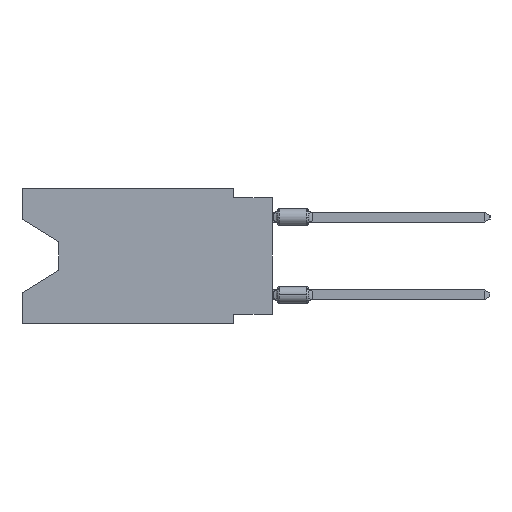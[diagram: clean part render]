
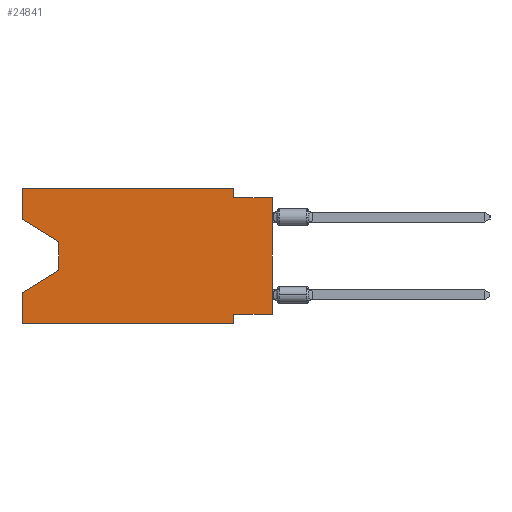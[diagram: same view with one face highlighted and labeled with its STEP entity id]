
A CAD part, left-side view. The second image highlights one B-rep face of the part: STEP entity #24841.
In plain terms, the highlighted planar face has unit normal (-1, 0, 0).
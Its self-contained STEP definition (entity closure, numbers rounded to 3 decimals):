
#209 = ORIENTED_EDGE ( 'NONE', *, *, #25861, .F. ) ;
#904 = VERTEX_POINT ( 'NONE', #20817 ) ;
#1866 = CARTESIAN_POINT ( 'NONE',  ( 0., 16.383, -8.89 ) ) ;
#4241 = CARTESIAN_POINT ( 'NONE',  ( 0., 13.97, -5.385 ) ) ;
#4389 = EDGE_CURVE ( 'NONE', #56818, #61978, #41734, .T. ) ;
#4486 = DIRECTION ( 'NONE',  ( 0., 0., -1. ) ) ;
#4579 = VECTOR ( 'NONE', #59693, 1000. ) ;
#4594 = VECTOR ( 'NONE', #38464, 1000. ) ;
#5525 = DIRECTION ( 'NONE',  ( 1., 0., 0. ) ) ;
#6193 = VECTOR ( 'NONE', #41860, 1000. ) ;
#6540 = VECTOR ( 'NONE', #58698, 1000. ) ;
#7580 = CARTESIAN_POINT ( 'NONE',  ( 0., 16.383, -6.852 ) ) ;
#8468 = VECTOR ( 'NONE', #64617, 1000. ) ;
#10137 = ORIENTED_EDGE ( 'NONE', *, *, #46131, .F. ) ;
#11813 = EDGE_CURVE ( 'NONE', #35556, #67885, #19351, .T. ) ;
#12263 = CARTESIAN_POINT ( 'NONE',  ( 0., 16.383, 0. ) ) ;
#12501 = VECTOR ( 'NONE', #23945, 1000. ) ;
#13232 = FACE_OUTER_BOUND ( 'NONE', #20999, .T. ) ;
#15757 = VERTEX_POINT ( 'NONE', #4241 ) ;
#15976 = CARTESIAN_POINT ( 'NONE',  ( 0., 16.383, -8.89 ) ) ;
#16066 = LINE ( 'NONE', #48453, #6193 ) ;
#17114 = EDGE_CURVE ( 'NONE', #15757, #41587, #45465, .T. ) ;
#17407 = EDGE_CURVE ( 'NONE', #61978, #28222, #37441, .T. ) ;
#17533 = CARTESIAN_POINT ( 'NONE',  ( 0., 13.97, -3.505 ) ) ;
#17977 = ORIENTED_EDGE ( 'NONE', *, *, #35410, .F. ) ;
#18123 = DIRECTION ( 'NONE',  ( 0., 0., 1. ) ) ;
#18981 = CARTESIAN_POINT ( 'NONE',  ( 0., 13.97, -5.385 ) ) ;
#19351 = LINE ( 'NONE', #20041, #64963 ) ;
#19603 = EDGE_CURVE ( 'NONE', #54139, #15757, #37781, .T. ) ;
#20041 = CARTESIAN_POINT ( 'NONE',  ( 0., 2.54, -8.89 ) ) ;
#20817 = CARTESIAN_POINT ( 'NONE',  ( 0., 16.383, -2.038 ) ) ;
#20999 = EDGE_LOOP ( 'NONE', ( #61478, #53809, #47068, #10137, #35614, #25546, #34554, #67553, #33373, #47545, #209, #17977 ) ) ;
#22217 = LINE ( 'NONE', #15976, #27086 ) ;
#23341 = CARTESIAN_POINT ( 'NONE',  ( 0., 16.383, 0. ) ) ;
#23405 = LINE ( 'NONE', #12263, #4579 ) ;
#23945 = DIRECTION ( 'NONE',  ( 0., 0., 1. ) ) ;
#24428 = VECTOR ( 'NONE', #49301, 1000. ) ;
#24841 = ADVANCED_FACE ( 'NONE', ( #13232 ), #34501, .F. ) ;
#25546 = ORIENTED_EDGE ( 'NONE', *, *, #11813, .F. ) ;
#25861 = EDGE_CURVE ( 'NONE', #46460, #56818, #27667, .T. ) ;
#26429 = VECTOR ( 'NONE', #62992, 1000. ) ;
#26431 = CARTESIAN_POINT ( 'NONE',  ( 0., 0., -0.635 ) ) ;
#27086 = VECTOR ( 'NONE', #38263, 1000. ) ;
#27667 = LINE ( 'NONE', #54495, #8468 ) ;
#28222 = VERTEX_POINT ( 'NONE', #26431 ) ;
#28438 = AXIS2_PLACEMENT_3D ( 'NONE', #47366, #5525, #4486 ) ;
#29304 = VERTEX_POINT ( 'NONE', #1866 ) ;
#29680 = CARTESIAN_POINT ( 'NONE',  ( 0., 13.97, -3.505 ) ) ;
#30039 = CARTESIAN_POINT ( 'NONE',  ( 0., 0., -8.255 ) ) ;
#30171 = EDGE_CURVE ( 'NONE', #52649, #28222, #50416, .T. ) ;
#30585 = CARTESIAN_POINT ( 'NONE',  ( 0., 2.54, 0. ) ) ;
#33373 = ORIENTED_EDGE ( 'NONE', *, *, #17407, .F. ) ;
#33531 = CARTESIAN_POINT ( 'NONE',  ( 0., 2.54, 0. ) ) ;
#34501 = PLANE ( 'NONE',  #28438 ) ;
#34554 = ORIENTED_EDGE ( 'NONE', *, *, #60709, .F. ) ;
#35410 = EDGE_CURVE ( 'NONE', #904, #46460, #23405, .T. ) ;
#35556 = VERTEX_POINT ( 'NONE', #62338 ) ;
#35614 = ORIENTED_EDGE ( 'NONE', *, *, #37666, .T. ) ;
#37237 = CARTESIAN_POINT ( 'NONE',  ( 0., 2.54, -8.89 ) ) ;
#37441 = LINE ( 'NONE', #68803, #6540 ) ;
#37666 = EDGE_CURVE ( 'NONE', #29304, #67885, #22217, .T. ) ;
#37713 = CARTESIAN_POINT ( 'NONE',  ( 0., 16.383, 0. ) ) ;
#37757 = CARTESIAN_POINT ( 'NONE',  ( 0., 2.54, -0.635 ) ) ;
#37781 = LINE ( 'NONE', #17533, #4594 ) ;
#38263 = DIRECTION ( 'NONE',  ( 0., -1., 0. ) ) ;
#38464 = DIRECTION ( 'NONE',  ( 0., 0., -1. ) ) ;
#38528 = CARTESIAN_POINT ( 'NONE',  ( 0., 0., -8.255 ) ) ;
#40431 = VECTOR ( 'NONE', #18123, 1000. ) ;
#41587 = VERTEX_POINT ( 'NONE', #7580 ) ;
#41734 = LINE ( 'NONE', #30585, #26429 ) ;
#41860 = DIRECTION ( 'NONE',  ( 0., -0.855, -0.519 ) ) ;
#43517 = EDGE_CURVE ( 'NONE', #904, #54139, #16066, .T. ) ;
#44269 = LINE ( 'NONE', #23341, #40431 ) ;
#44786 = DIRECTION ( 'NONE',  ( 0., 0.855, -0.519 ) ) ;
#45465 = LINE ( 'NONE', #18981, #55544 ) ;
#46131 = EDGE_CURVE ( 'NONE', #29304, #41587, #44269, .T. ) ;
#46460 = VERTEX_POINT ( 'NONE', #37713 ) ;
#47068 = ORIENTED_EDGE ( 'NONE', *, *, #17114, .T. ) ;
#47366 = CARTESIAN_POINT ( 'NONE',  ( 0., 16.383, 0. ) ) ;
#47545 = ORIENTED_EDGE ( 'NONE', *, *, #4389, .F. ) ;
#48453 = CARTESIAN_POINT ( 'NONE',  ( 0., 16.383, -2.038 ) ) ;
#49301 = DIRECTION ( 'NONE',  ( 0., 1., 0. ) ) ;
#50416 = LINE ( 'NONE', #60216, #12501 ) ;
#52649 = VERTEX_POINT ( 'NONE', #30039 ) ;
#53809 = ORIENTED_EDGE ( 'NONE', *, *, #19603, .T. ) ;
#54139 = VERTEX_POINT ( 'NONE', #29680 ) ;
#54495 = CARTESIAN_POINT ( 'NONE',  ( 0., 16.383, 0. ) ) ;
#55544 = VECTOR ( 'NONE', #44786, 1000. ) ;
#56818 = VERTEX_POINT ( 'NONE', #33531 ) ;
#58698 = DIRECTION ( 'NONE',  ( 0., -1., 0. ) ) ;
#59446 = LINE ( 'NONE', #38528, #24428 ) ;
#59693 = DIRECTION ( 'NONE',  ( 0., 0., 1. ) ) ;
#60216 = CARTESIAN_POINT ( 'NONE',  ( 0., 0., 0. ) ) ;
#60709 = EDGE_CURVE ( 'NONE', #52649, #35556, #59446, .T. ) ;
#61478 = ORIENTED_EDGE ( 'NONE', *, *, #43517, .T. ) ;
#61978 = VERTEX_POINT ( 'NONE', #37757 ) ;
#62338 = CARTESIAN_POINT ( 'NONE',  ( 0., 2.54, -8.255 ) ) ;
#62913 = DIRECTION ( 'NONE',  ( 0., 0., -1. ) ) ;
#62992 = DIRECTION ( 'NONE',  ( 0., 0., -1. ) ) ;
#64617 = DIRECTION ( 'NONE',  ( 0., -1., 0. ) ) ;
#64963 = VECTOR ( 'NONE', #62913, 1000. ) ;
#67553 = ORIENTED_EDGE ( 'NONE', *, *, #30171, .T. ) ;
#67885 = VERTEX_POINT ( 'NONE', #37237 ) ;
#68803 = CARTESIAN_POINT ( 'NONE',  ( 0., 0., -0.635 ) ) ;
